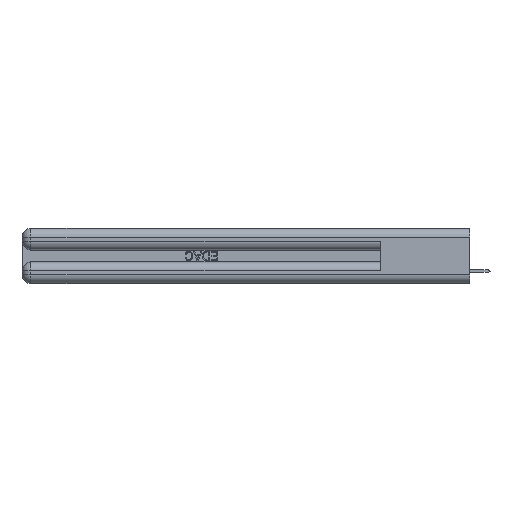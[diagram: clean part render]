
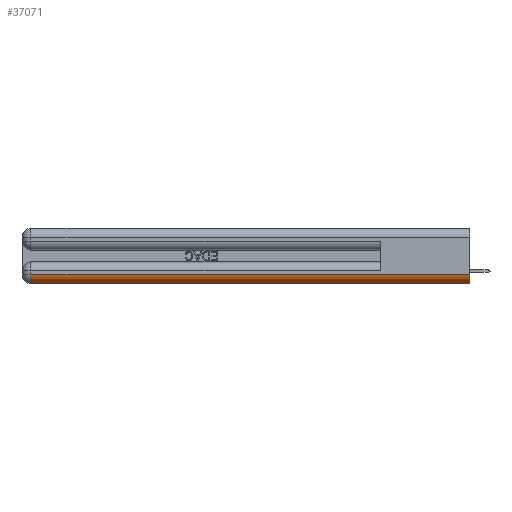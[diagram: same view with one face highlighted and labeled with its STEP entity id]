
A CAD part, left-side view. The second image highlights one B-rep face of the part: STEP entity #37071.
In plain terms, the highlighted cylindrical face has radius 1.524 mm (diameter 3.048 mm), a partial arc.
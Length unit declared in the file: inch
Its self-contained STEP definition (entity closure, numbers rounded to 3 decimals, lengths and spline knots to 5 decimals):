
#467 = CARTESIAN_POINT ( 'NONE',  ( 0., 0., 0.06 ) ) ;
#2982 = CARTESIAN_POINT ( 'NONE',  ( 0.06, 2.94, 0.06 ) ) ;
#3257 = DIRECTION ( 'NONE',  ( 0., 0., 1. ) ) ;
#3421 = CARTESIAN_POINT ( 'NONE',  ( 0., 2.94, 0.06 ) ) ;
#4982 = VECTOR ( 'NONE', #25826, 39.37008 ) ;
#5660 = LINE ( 'NONE', #25309, #4982 ) ;
#6447 = AXIS2_PLACEMENT_3D ( 'NONE', #51073, #31427, #3257 ) ;
#9912 = DIRECTION ( 'NONE',  ( 0., 0., 1. ) ) ;
#11785 = EDGE_LOOP ( 'NONE', ( #34005, #24940, #15935, #42761 ) ) ;
#11807 = CIRCLE ( 'NONE', #29133, 0.06 ) ;
#11974 = EDGE_CURVE ( 'NONE', #49567, #15353, #30401, .T. ) ;
#15353 = VERTEX_POINT ( 'NONE', #29525 ) ;
#15449 = CARTESIAN_POINT ( 'NONE',  ( 0.06, 2.94, 0. ) ) ;
#15566 = LINE ( 'NONE', #18936, #28273 ) ;
#15920 = EDGE_CURVE ( 'NONE', #18861, #49567, #5660, .T. ) ;
#15935 = ORIENTED_EDGE ( 'NONE', *, *, #18241, .F. ) ;
#17646 = CYLINDRICAL_SURFACE ( 'NONE', #34737, 0.06 ) ;
#18183 = DIRECTION ( 'NONE',  ( 0., 1., 0. ) ) ;
#18241 = EDGE_CURVE ( 'NONE', #26350, #18861, #11807, .T. ) ;
#18861 = VERTEX_POINT ( 'NONE', #3421 ) ;
#18936 = CARTESIAN_POINT ( 'NONE',  ( 0.06, 3., 0. ) ) ;
#24940 = ORIENTED_EDGE ( 'NONE', *, *, #15920, .F. ) ;
#25309 = CARTESIAN_POINT ( 'NONE',  ( 0., 0., 0.06 ) ) ;
#25826 = DIRECTION ( 'NONE',  ( 0., -1., 0. ) ) ;
#26225 = DIRECTION ( 'NONE',  ( 0., 0., 1. ) ) ;
#26350 = VERTEX_POINT ( 'NONE', #15449 ) ;
#26726 = DIRECTION ( 'NONE',  ( 0., 1., 0. ) ) ;
#28273 = VECTOR ( 'NONE', #26726, 39.37008 ) ;
#29133 = AXIS2_PLACEMENT_3D ( 'NONE', #2982, #18183, #26225 ) ;
#29525 = CARTESIAN_POINT ( 'NONE',  ( 0.06, 0., 0. ) ) ;
#29587 = CARTESIAN_POINT ( 'NONE',  ( 0.06, 0., 0.06 ) ) ;
#30401 = CIRCLE ( 'NONE', #6447, 0.06 ) ;
#31427 = DIRECTION ( 'NONE',  ( 0., -1., 0. ) ) ;
#34005 = ORIENTED_EDGE ( 'NONE', *, *, #11974, .F. ) ;
#34737 = AXIS2_PLACEMENT_3D ( 'NONE', #29587, #45371, #9912 ) ;
#37071 = ADVANCED_FACE ( 'NONE', ( #41495 ), #17646, .T. ) ;
#41495 = FACE_OUTER_BOUND ( 'NONE', #11785, .T. ) ;
#42761 = ORIENTED_EDGE ( 'NONE', *, *, #49928, .F. ) ;
#45371 = DIRECTION ( 'NONE',  ( 0., 1., 0. ) ) ;
#49567 = VERTEX_POINT ( 'NONE', #467 ) ;
#49928 = EDGE_CURVE ( 'NONE', #15353, #26350, #15566, .T. ) ;
#51073 = CARTESIAN_POINT ( 'NONE',  ( 0.06, 0., 0.06 ) ) ;
